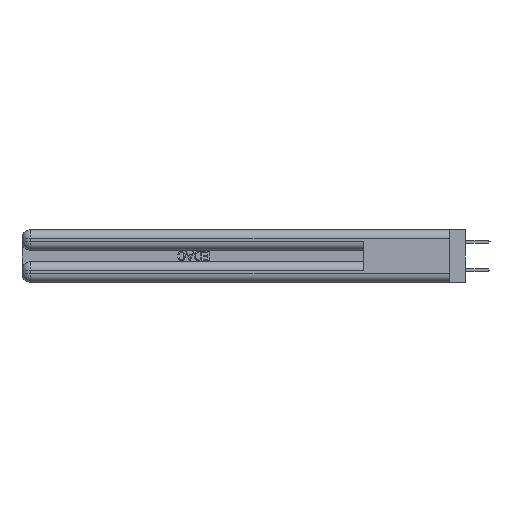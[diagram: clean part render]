
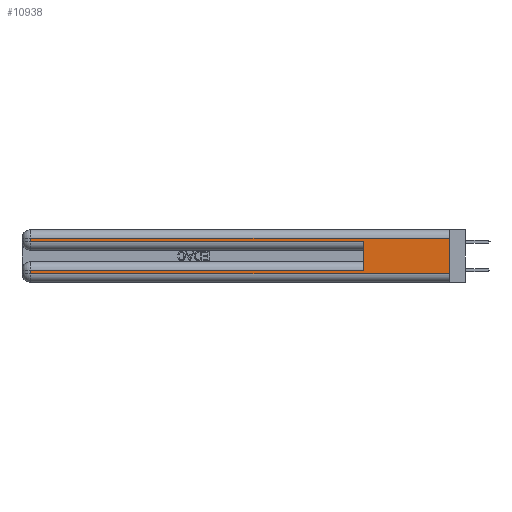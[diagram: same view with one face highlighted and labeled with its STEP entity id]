
A CAD part, left-side view. The second image highlights one B-rep face of the part: STEP entity #10938.
In plain terms, the highlighted planar face has unit normal (-1, 0, 0).
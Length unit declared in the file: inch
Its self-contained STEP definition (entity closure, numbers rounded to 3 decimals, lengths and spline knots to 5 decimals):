
#103 = VECTOR ( 'NONE', #37526, 39.37008 ) ;
#111 = PLANE ( 'NONE',  #37079 ) ;
#265 = VERTEX_POINT ( 'NONE', #31426 ) ;
#473 = CARTESIAN_POINT ( 'NONE',  ( 0., 2.94, 0.37 ) ) ;
#787 = EDGE_CURVE ( 'NONE', #265, #18906, #32730, .T. ) ;
#1705 = CARTESIAN_POINT ( 'NONE',  ( 0., 0., 0.37 ) ) ;
#2303 = EDGE_CURVE ( 'NONE', #26916, #14172, #26668, .T. ) ;
#2309 = DIRECTION ( 'NONE',  ( 0., -1., 0. ) ) ;
#2690 = EDGE_CURVE ( 'NONE', #30844, #26916, #20353, .T. ) ;
#3701 = ORIENTED_EDGE ( 'NONE', *, *, #2303, .T. ) ;
#4438 = FACE_OUTER_BOUND ( 'NONE', #20366, .T. ) ;
#6253 = VERTEX_POINT ( 'NONE', #37658 ) ;
#6844 = VECTOR ( 'NONE', #27960, 39.37008 ) ;
#7504 = VECTOR ( 'NONE', #12379, 39.37008 ) ;
#7543 = LINE ( 'NONE', #1705, #15645 ) ;
#8265 = LINE ( 'NONE', #8534, #41411 ) ;
#8534 = CARTESIAN_POINT ( 'NONE',  ( 0., 0., 0.31 ) ) ;
#10518 = LINE ( 'NONE', #15313, #37770 ) ;
#10683 = EDGE_CURVE ( 'NONE', #30427, #14172, #43499, .T. ) ;
#10938 = ADVANCED_FACE ( 'NONE', ( #4438 ), #111, .F. ) ;
#11409 = CARTESIAN_POINT ( 'NONE',  ( 0., 0.6, 0.285 ) ) ;
#12379 = DIRECTION ( 'NONE',  ( 0., 1., 0. ) ) ;
#13068 = ORIENTED_EDGE ( 'NONE', *, *, #10683, .F. ) ;
#14051 = DIRECTION ( 'NONE',  ( 0., 0., -1. ) ) ;
#14172 = VERTEX_POINT ( 'NONE', #11409 ) ;
#14908 = VERTEX_POINT ( 'NONE', #38772 ) ;
#15313 = CARTESIAN_POINT ( 'NONE',  ( 0., 0., 0.06 ) ) ;
#15645 = VECTOR ( 'NONE', #25470, 39.37008 ) ;
#16915 = ORIENTED_EDGE ( 'NONE', *, *, #787, .T. ) ;
#18906 = VERTEX_POINT ( 'NONE', #29461 ) ;
#20353 = LINE ( 'NONE', #473, #6844 ) ;
#20366 = EDGE_LOOP ( 'NONE', ( #35667, #36638, #23804, #3701, #13068, #30864, #16915, #37275 ) ) ;
#22797 = CARTESIAN_POINT ( 'NONE',  ( 0., 2.94, 0.31 ) ) ;
#22855 = CARTESIAN_POINT ( 'NONE',  ( 0., 0., 0.085 ) ) ;
#23214 = VECTOR ( 'NONE', #27365, 39.37008 ) ;
#23417 = EDGE_CURVE ( 'NONE', #14908, #6253, #7543, .T. ) ;
#23804 = ORIENTED_EDGE ( 'NONE', *, *, #2690, .T. ) ;
#25470 = DIRECTION ( 'NONE',  ( 0., 0., -1. ) ) ;
#26668 = LINE ( 'NONE', #36585, #38439 ) ;
#26916 = VERTEX_POINT ( 'NONE', #37998 ) ;
#27271 = EDGE_CURVE ( 'NONE', #14908, #30844, #8265, .T. ) ;
#27365 = DIRECTION ( 'NONE',  ( 0., 0., 1. ) ) ;
#27960 = DIRECTION ( 'NONE',  ( 0., 0., -1. ) ) ;
#29461 = CARTESIAN_POINT ( 'NONE',  ( 0., 2.94, 0.06 ) ) ;
#30427 = VERTEX_POINT ( 'NONE', #34133 ) ;
#30798 = CARTESIAN_POINT ( 'NONE',  ( 0., 2.94, 0.37 ) ) ;
#30844 = VERTEX_POINT ( 'NONE', #22797 ) ;
#30864 = ORIENTED_EDGE ( 'NONE', *, *, #37659, .T. ) ;
#31406 = EDGE_CURVE ( 'NONE', #18906, #6253, #10518, .T. ) ;
#31426 = CARTESIAN_POINT ( 'NONE',  ( 0., 2.94, 0.085 ) ) ;
#32730 = LINE ( 'NONE', #30798, #103 ) ;
#34099 = CARTESIAN_POINT ( 'NONE',  ( 0., 0.6, 0.145 ) ) ;
#34133 = CARTESIAN_POINT ( 'NONE',  ( 0., 0.6, 0.085 ) ) ;
#34807 = LINE ( 'NONE', #22855, #7504 ) ;
#35667 = ORIENTED_EDGE ( 'NONE', *, *, #23417, .F. ) ;
#36585 = CARTESIAN_POINT ( 'NONE',  ( 0., 0., 0.285 ) ) ;
#36638 = ORIENTED_EDGE ( 'NONE', *, *, #27271, .T. ) ;
#37079 = AXIS2_PLACEMENT_3D ( 'NONE', #38206, #41925, #14051 ) ;
#37275 = ORIENTED_EDGE ( 'NONE', *, *, #31406, .T. ) ;
#37526 = DIRECTION ( 'NONE',  ( 0., 0., -1. ) ) ;
#37658 = CARTESIAN_POINT ( 'NONE',  ( 0., 0., 0.06 ) ) ;
#37659 = EDGE_CURVE ( 'NONE', #30427, #265, #34807, .T. ) ;
#37770 = VECTOR ( 'NONE', #42427, 39.37008 ) ;
#37998 = CARTESIAN_POINT ( 'NONE',  ( 0., 2.94, 0.285 ) ) ;
#38206 = CARTESIAN_POINT ( 'NONE',  ( 0., 0., 0.37 ) ) ;
#38439 = VECTOR ( 'NONE', #2309, 39.37008 ) ;
#38772 = CARTESIAN_POINT ( 'NONE',  ( 0., 0., 0.31 ) ) ;
#41411 = VECTOR ( 'NONE', #42900, 39.37008 ) ;
#41925 = DIRECTION ( 'NONE',  ( 1., 0., 0. ) ) ;
#42427 = DIRECTION ( 'NONE',  ( 0., -1., 0. ) ) ;
#42900 = DIRECTION ( 'NONE',  ( 0., 1., 0. ) ) ;
#43499 = LINE ( 'NONE', #34099, #23214 ) ;
